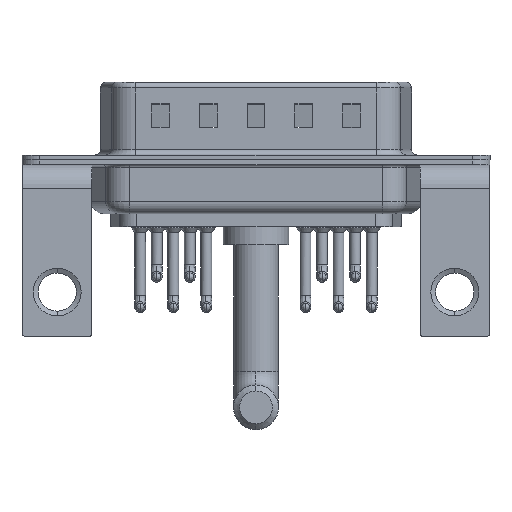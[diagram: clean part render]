
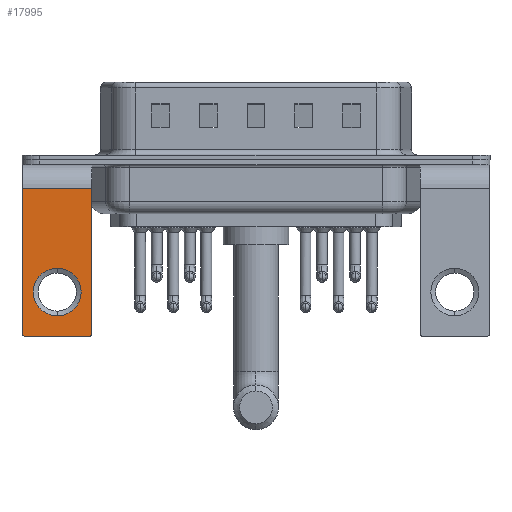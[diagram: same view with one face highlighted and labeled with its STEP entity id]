
A CAD part, front view. The second image highlights one B-rep face of the part: STEP entity #17995.
In plain terms, the highlighted planar face has unit normal (0, -1, 0).
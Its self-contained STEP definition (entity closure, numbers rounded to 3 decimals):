
#122 = CARTESIAN_POINT ( 'NONE',  ( -2.9, -6.25, -2.4 ) ) ;
#182 = CARTESIAN_POINT ( 'NONE',  ( -2.9, -6.25, -14.55 ) ) ;
#207 = VERTEX_POINT ( 'NONE', #3453 ) ;
#430 = ORIENTED_EDGE ( 'NONE', *, *, #19795, .F. ) ;
#570 = CIRCLE ( 'NONE', #16625, 0.25 ) ;
#890 = AXIS2_PLACEMENT_3D ( 'NONE', #7988, #11377, #7872 ) ;
#2171 = LINE ( 'NONE', #21624, #5536 ) ;
#2189 = CARTESIAN_POINT ( 'NONE',  ( 0., -6.25, -11.07 ) ) ;
#2299 = CARTESIAN_POINT ( 'NONE',  ( 2.65, -6.25, -14.55 ) ) ;
#2510 = VERTEX_POINT ( 'NONE', #122 ) ;
#3286 = DIRECTION ( 'NONE',  ( 0., 0., 1. ) ) ;
#3453 = CARTESIAN_POINT ( 'NONE',  ( 0., -6.25, -9.07 ) ) ;
#3724 = VERTEX_POINT ( 'NONE', #8211 ) ;
#4229 = CIRCLE ( 'NONE', #19929, 2. ) ;
#4240 = FACE_BOUND ( 'NONE', #21950, .T. ) ;
#5022 = LINE ( 'NONE', #22678, #10190 ) ;
#5208 = DIRECTION ( 'NONE',  ( 0., 1., 0. ) ) ;
#5467 = DIRECTION ( 'NONE',  ( 0., 0., -1. ) ) ;
#5536 = VECTOR ( 'NONE', #5467, 1000. ) ;
#5801 = DIRECTION ( 'NONE',  ( -1., 0., 0. ) ) ;
#5943 = VERTEX_POINT ( 'NONE', #13422 ) ;
#5959 = EDGE_CURVE ( 'NONE', #17654, #21709, #570, .T. ) ;
#6162 = VERTEX_POINT ( 'NONE', #182 ) ;
#6772 = DIRECTION ( 'NONE',  ( 0., 0., -1. ) ) ;
#7259 = DIRECTION ( 'NONE',  ( 0., -1., 0. ) ) ;
#7677 = VECTOR ( 'NONE', #20505, 1000. ) ;
#7872 = DIRECTION ( 'NONE',  ( 0., 0., 1. ) ) ;
#7988 = CARTESIAN_POINT ( 'NONE',  ( 2.9, -6.25, -2.4 ) ) ;
#7997 = CIRCLE ( 'NONE', #19183, 2. ) ;
#8211 = CARTESIAN_POINT ( 'NONE',  ( 2.9, -6.25, -2.4 ) ) ;
#8346 = CARTESIAN_POINT ( 'NONE',  ( 0., -6.25, -11.07 ) ) ;
#8452 = EDGE_CURVE ( 'NONE', #2510, #6162, #2171, .T. ) ;
#8688 = DIRECTION ( 'NONE',  ( 0., 0., 1. ) ) ;
#8865 = EDGE_LOOP ( 'NONE', ( #12135, #10193, #430, #18997, #9725, #11546 ) ) ;
#9725 = ORIENTED_EDGE ( 'NONE', *, *, #16297, .F. ) ;
#10190 = VECTOR ( 'NONE', #6772, 1000. ) ;
#10193 = ORIENTED_EDGE ( 'NONE', *, *, #11358, .T. ) ;
#11358 = EDGE_CURVE ( 'NONE', #6162, #5943, #19399, .T. ) ;
#11377 = DIRECTION ( 'NONE',  ( 0., 1., 0. ) ) ;
#11546 = ORIENTED_EDGE ( 'NONE', *, *, #15362, .T. ) ;
#11989 = CARTESIAN_POINT ( 'NONE',  ( 2.65, -6.25, -14.8 ) ) ;
#12135 = ORIENTED_EDGE ( 'NONE', *, *, #8452, .T. ) ;
#12310 = CARTESIAN_POINT ( 'NONE',  ( -2.65, -6.25, -14.55 ) ) ;
#12534 = VERTEX_POINT ( 'NONE', #15801 ) ;
#12568 = ORIENTED_EDGE ( 'NONE', *, *, #18124, .T. ) ;
#12955 = DIRECTION ( 'NONE',  ( 0., 1., 0. ) ) ;
#13303 = DIRECTION ( 'NONE',  ( 0., 0., 1. ) ) ;
#13422 = CARTESIAN_POINT ( 'NONE',  ( -2.65, -6.25, -14.8 ) ) ;
#15326 = CARTESIAN_POINT ( 'NONE',  ( 2.9, -6.25, -14.55 ) ) ;
#15362 = EDGE_CURVE ( 'NONE', #3724, #2510, #20199, .T. ) ;
#15801 = CARTESIAN_POINT ( 'NONE',  ( 0., -6.25, -13.07 ) ) ;
#16135 = VECTOR ( 'NONE', #5801, 1000. ) ;
#16297 = EDGE_CURVE ( 'NONE', #3724, #21709, #5022, .T. ) ;
#16625 = AXIS2_PLACEMENT_3D ( 'NONE', #2299, #20564, #13303 ) ;
#16747 = LINE ( 'NONE', #20382, #7677 ) ;
#17533 = AXIS2_PLACEMENT_3D ( 'NONE', #12310, #7259, #3286 ) ;
#17638 = EDGE_CURVE ( 'NONE', #207, #12534, #4229, .T. ) ;
#17654 = VERTEX_POINT ( 'NONE', #11989 ) ;
#17995 = ADVANCED_FACE ( 'NONE', ( #4240, #18389 ), #20270, .F. ) ;
#18124 = EDGE_CURVE ( 'NONE', #12534, #207, #7997, .T. ) ;
#18389 = FACE_OUTER_BOUND ( 'NONE', #8865, .T. ) ;
#18938 = ORIENTED_EDGE ( 'NONE', *, *, #17638, .T. ) ;
#18997 = ORIENTED_EDGE ( 'NONE', *, *, #5959, .T. ) ;
#19183 = AXIS2_PLACEMENT_3D ( 'NONE', #2189, #12955, #20210 ) ;
#19399 = CIRCLE ( 'NONE', #17533, 0.25 ) ;
#19795 = EDGE_CURVE ( 'NONE', #17654, #5943, #16747, .T. ) ;
#19929 = AXIS2_PLACEMENT_3D ( 'NONE', #8346, #5208, #8688 ) ;
#20199 = LINE ( 'NONE', #21842, #16135 ) ;
#20210 = DIRECTION ( 'NONE',  ( 0., 0., 1. ) ) ;
#20270 = PLANE ( 'NONE',  #890 ) ;
#20382 = CARTESIAN_POINT ( 'NONE',  ( 2.9, -6.25, -14.8 ) ) ;
#20505 = DIRECTION ( 'NONE',  ( -1., 0., 0. ) ) ;
#20564 = DIRECTION ( 'NONE',  ( 0., -1., 0. ) ) ;
#21624 = CARTESIAN_POINT ( 'NONE',  ( -2.9, -6.25, -2.4 ) ) ;
#21709 = VERTEX_POINT ( 'NONE', #15326 ) ;
#21842 = CARTESIAN_POINT ( 'NONE',  ( 2.9, -6.25, -2.4 ) ) ;
#21950 = EDGE_LOOP ( 'NONE', ( #12568, #18938 ) ) ;
#22678 = CARTESIAN_POINT ( 'NONE',  ( 2.9, -6.25, -2.4 ) ) ;
